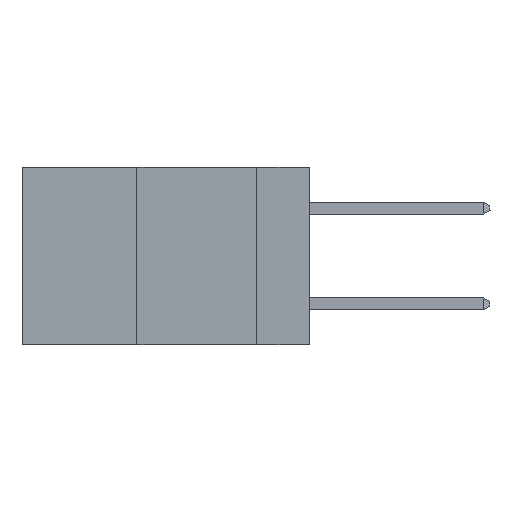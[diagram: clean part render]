
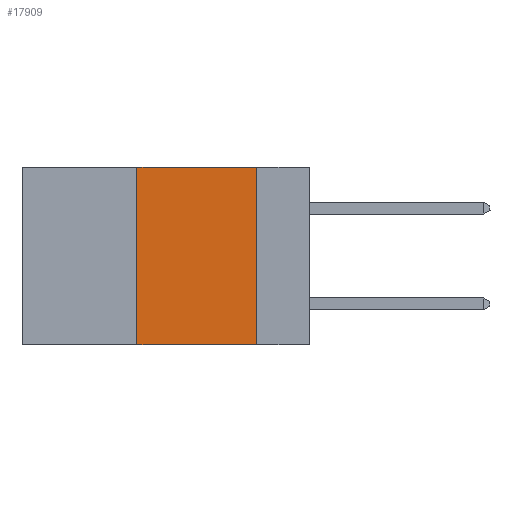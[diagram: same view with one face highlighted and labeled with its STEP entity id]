
A CAD part, left-side view. The second image highlights one B-rep face of the part: STEP entity #17909.
In plain terms, the highlighted planar face has unit normal (-1, 0, 0).
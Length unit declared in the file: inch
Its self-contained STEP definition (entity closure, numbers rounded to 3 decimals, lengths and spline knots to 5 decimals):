
#76 = FACE_OUTER_BOUND ( 'NONE', #20662, .T. ) ;
#2902 = VERTEX_POINT ( 'NONE', #38294 ) ;
#4798 = CARTESIAN_POINT ( 'NONE',  ( 0., 0.11, 0. ) ) ;
#6910 = EDGE_CURVE ( 'NONE', #31327, #16013, #20282, .T. ) ;
#8241 = VECTOR ( 'NONE', #36333, 39.37008 ) ;
#13420 = AXIS2_PLACEMENT_3D ( 'NONE', #27060, #24808, #39814 ) ;
#13955 = EDGE_CURVE ( 'NONE', #16013, #18704, #27617, .T. ) ;
#16013 = VERTEX_POINT ( 'NONE', #35049 ) ;
#17172 = DIRECTION ( 'NONE',  ( 0., 0., -1. ) ) ;
#17909 = ADVANCED_FACE ( 'NONE', ( #76 ), #33738, .F. ) ;
#18523 = ORIENTED_EDGE ( 'NONE', *, *, #32156, .T. ) ;
#18704 = VERTEX_POINT ( 'NONE', #24545 ) ;
#19512 = CARTESIAN_POINT ( 'NONE',  ( 0., 0.36, -0.37 ) ) ;
#20282 = LINE ( 'NONE', #33449, #29390 ) ;
#20662 = EDGE_LOOP ( 'NONE', ( #30638, #32435, #21498, #18523 ) ) ;
#20850 = LINE ( 'NONE', #27349, #39819 ) ;
#21498 = ORIENTED_EDGE ( 'NONE', *, *, #6910, .F. ) ;
#24545 = CARTESIAN_POINT ( 'NONE',  ( 0., 0.11, 0. ) ) ;
#24808 = DIRECTION ( 'NONE',  ( 1., 0., 0. ) ) ;
#27060 = CARTESIAN_POINT ( 'NONE',  ( 0., 0.6, 0. ) ) ;
#27349 = CARTESIAN_POINT ( 'NONE',  ( 0., 0.6, -0.37 ) ) ;
#27617 = LINE ( 'NONE', #39973, #8241 ) ;
#29390 = VECTOR ( 'NONE', #32657, 39.37008 ) ;
#29763 = EDGE_CURVE ( 'NONE', #18704, #2902, #39257, .T. ) ;
#30638 = ORIENTED_EDGE ( 'NONE', *, *, #29763, .F. ) ;
#31327 = VERTEX_POINT ( 'NONE', #19512 ) ;
#32156 = EDGE_CURVE ( 'NONE', #31327, #2902, #20850, .T. ) ;
#32435 = ORIENTED_EDGE ( 'NONE', *, *, #13955, .F. ) ;
#32657 = DIRECTION ( 'NONE',  ( 0., 0., 1. ) ) ;
#33199 = VECTOR ( 'NONE', #17172, 39.37008 ) ;
#33449 = CARTESIAN_POINT ( 'NONE',  ( 0., 0.36, 0. ) ) ;
#33738 = PLANE ( 'NONE',  #13420 ) ;
#35049 = CARTESIAN_POINT ( 'NONE',  ( 0., 0.36, 0. ) ) ;
#36333 = DIRECTION ( 'NONE',  ( 0., -1., 0. ) ) ;
#36462 = DIRECTION ( 'NONE',  ( 0., -1., 0. ) ) ;
#38294 = CARTESIAN_POINT ( 'NONE',  ( 0., 0.11, -0.37 ) ) ;
#39257 = LINE ( 'NONE', #4798, #33199 ) ;
#39814 = DIRECTION ( 'NONE',  ( 0., 0., -1. ) ) ;
#39819 = VECTOR ( 'NONE', #36462, 39.37008 ) ;
#39973 = CARTESIAN_POINT ( 'NONE',  ( 0., 0.6, 0. ) ) ;
